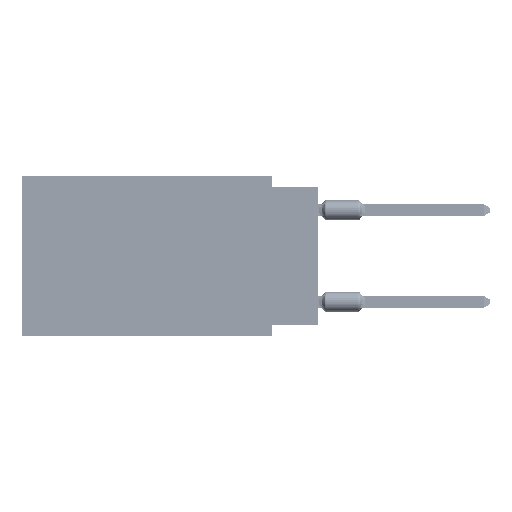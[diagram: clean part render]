
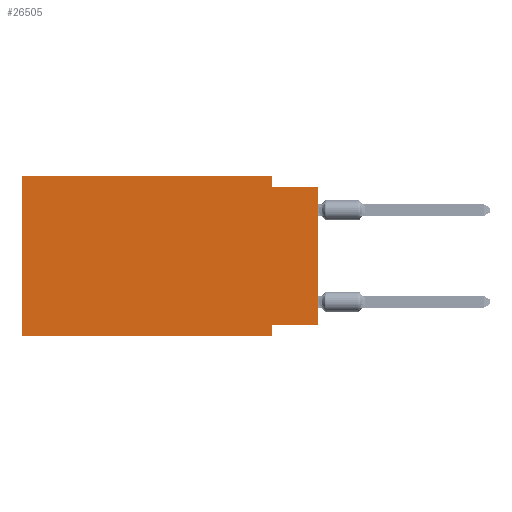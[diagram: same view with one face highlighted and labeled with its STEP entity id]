
A CAD part, left-side view. The second image highlights one B-rep face of the part: STEP entity #26505.
In plain terms, the highlighted planar face has unit normal (-1, 0, 0).
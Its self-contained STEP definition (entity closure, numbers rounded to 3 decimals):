
#7209 = FACE_OUTER_BOUND ( 'NONE', #78304, .T. ) ;
#9308 = EDGE_CURVE ( 'NONE', #32123, #52442, #19583, .T. ) ;
#13279 = ORIENTED_EDGE ( 'NONE', *, *, #82585, .F. ) ;
#13692 = ORIENTED_EDGE ( 'NONE', *, *, #56517, .T. ) ;
#13972 = DIRECTION ( 'NONE',  ( 0., 0., -1. ) ) ;
#15621 = VECTOR ( 'NONE', #25008, 1000. ) ;
#16963 = VECTOR ( 'NONE', #35769, 1000. ) ;
#17508 = EDGE_CURVE ( 'NONE', #52442, #57949, #81230, .T. ) ;
#18254 = EDGE_CURVE ( 'NONE', #26340, #76185, #29780, .T. ) ;
#19583 = LINE ( 'NONE', #56769, #20779 ) ;
#20358 = CARTESIAN_POINT ( 'NONE',  ( 0., 2.54, -8.255 ) ) ;
#20393 = LINE ( 'NONE', #85616, #67658 ) ;
#20779 = VECTOR ( 'NONE', #62588, 1000. ) ;
#25008 = DIRECTION ( 'NONE',  ( 0., 0., 1. ) ) ;
#26340 = VERTEX_POINT ( 'NONE', #94135 ) ;
#26505 = ADVANCED_FACE ( 'NONE', ( #7209 ), #37137, .F. ) ;
#26894 = AXIS2_PLACEMENT_3D ( 'NONE', #36192, #50203, #13972 ) ;
#28826 = CARTESIAN_POINT ( 'NONE',  ( 0., 0., -0.635 ) ) ;
#29326 = CARTESIAN_POINT ( 'NONE',  ( 0., 16.383, 0. ) ) ;
#29780 = LINE ( 'NONE', #28826, #38343 ) ;
#30256 = DIRECTION ( 'NONE',  ( 0., -1., 0. ) ) ;
#32123 = VERTEX_POINT ( 'NONE', #59922 ) ;
#32462 = CARTESIAN_POINT ( 'NONE',  ( 0., 2.54, -8.89 ) ) ;
#35296 = LINE ( 'NONE', #86037, #16963 ) ;
#35614 = LINE ( 'NONE', #29326, #61478 ) ;
#35769 = DIRECTION ( 'NONE',  ( 0., 0., -1. ) ) ;
#36192 = CARTESIAN_POINT ( 'NONE',  ( 0., 16.383, 0. ) ) ;
#36251 = ORIENTED_EDGE ( 'NONE', *, *, #17508, .F. ) ;
#37137 = PLANE ( 'NONE',  #26894 ) ;
#38343 = VECTOR ( 'NONE', #30256, 1000. ) ;
#39496 = CARTESIAN_POINT ( 'NONE',  ( 0., 0., 0. ) ) ;
#39823 = EDGE_CURVE ( 'NONE', #32123, #76185, #75731, .T. ) ;
#42604 = VERTEX_POINT ( 'NONE', #52456 ) ;
#43943 = ORIENTED_EDGE ( 'NONE', *, *, #9308, .F. ) ;
#45443 = CARTESIAN_POINT ( 'NONE',  ( 0., 2.54, -8.89 ) ) ;
#49836 = DIRECTION ( 'NONE',  ( 0., 0., 1. ) ) ;
#50203 = DIRECTION ( 'NONE',  ( 1., 0., 0. ) ) ;
#52442 = VERTEX_POINT ( 'NONE', #20358 ) ;
#52456 = CARTESIAN_POINT ( 'NONE',  ( 0., 2.54, 0. ) ) ;
#54529 = CARTESIAN_POINT ( 'NONE',  ( 0., 16.383, -8.89 ) ) ;
#56517 = EDGE_CURVE ( 'NONE', #59545, #57949, #78896, .T. ) ;
#56769 = CARTESIAN_POINT ( 'NONE',  ( 0., 0., -8.255 ) ) ;
#57012 = CARTESIAN_POINT ( 'NONE',  ( 0., 0., -0.635 ) ) ;
#57949 = VERTEX_POINT ( 'NONE', #32462 ) ;
#58229 = EDGE_CURVE ( 'NONE', #42604, #26340, #35296, .T. ) ;
#59545 = VERTEX_POINT ( 'NONE', #54529 ) ;
#59922 = CARTESIAN_POINT ( 'NONE',  ( 0., 0., -8.255 ) ) ;
#61478 = VECTOR ( 'NONE', #81025, 1000. ) ;
#61985 = VERTEX_POINT ( 'NONE', #83180 ) ;
#62588 = DIRECTION ( 'NONE',  ( 0., 1., 0. ) ) ;
#62944 = ORIENTED_EDGE ( 'NONE', *, *, #39823, .T. ) ;
#63432 = CARTESIAN_POINT ( 'NONE',  ( 0., 16.383, -8.89 ) ) ;
#67658 = VECTOR ( 'NONE', #49836, 1000. ) ;
#69065 = VECTOR ( 'NONE', #72582, 1000. ) ;
#72582 = DIRECTION ( 'NONE',  ( 0., -1., 0. ) ) ;
#75172 = VECTOR ( 'NONE', #88464, 1000. ) ;
#75731 = LINE ( 'NONE', #39496, #15621 ) ;
#76185 = VERTEX_POINT ( 'NONE', #57012 ) ;
#77806 = ORIENTED_EDGE ( 'NONE', *, *, #95295, .F. ) ;
#78304 = EDGE_LOOP ( 'NONE', ( #62944, #78345, #92120, #77806, #13279, #13692, #36251, #43943 ) ) ;
#78345 = ORIENTED_EDGE ( 'NONE', *, *, #18254, .F. ) ;
#78896 = LINE ( 'NONE', #63432, #69065 ) ;
#81025 = DIRECTION ( 'NONE',  ( 0., -1., 0. ) ) ;
#81230 = LINE ( 'NONE', #45443, #75172 ) ;
#82585 = EDGE_CURVE ( 'NONE', #59545, #61985, #20393, .T. ) ;
#83180 = CARTESIAN_POINT ( 'NONE',  ( 0., 16.383, 0. ) ) ;
#85616 = CARTESIAN_POINT ( 'NONE',  ( 0., 16.383, 0. ) ) ;
#86037 = CARTESIAN_POINT ( 'NONE',  ( 0., 2.54, 0. ) ) ;
#88464 = DIRECTION ( 'NONE',  ( 0., 0., -1. ) ) ;
#92120 = ORIENTED_EDGE ( 'NONE', *, *, #58229, .F. ) ;
#94135 = CARTESIAN_POINT ( 'NONE',  ( 0., 2.54, -0.635 ) ) ;
#95295 = EDGE_CURVE ( 'NONE', #61985, #42604, #35614, .T. ) ;
